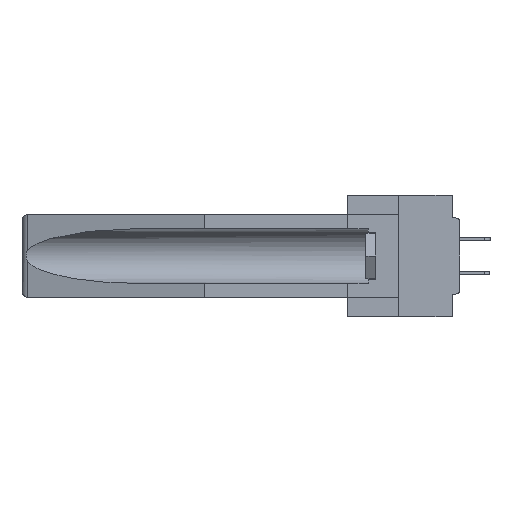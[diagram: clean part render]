
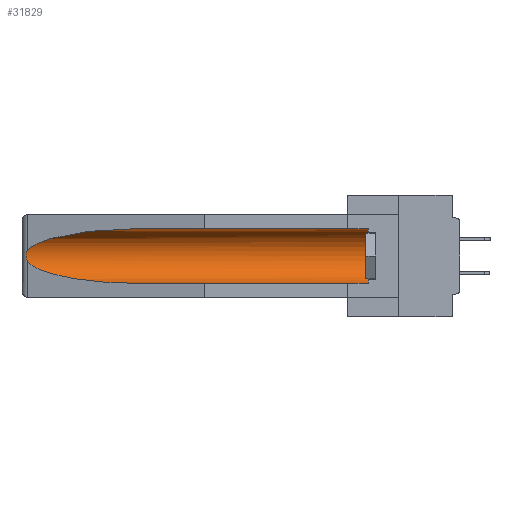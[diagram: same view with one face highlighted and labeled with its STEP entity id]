
A CAD part, left-side view. The second image highlights one B-rep face of the part: STEP entity #31829.
In plain terms, the highlighted cylindrical face has radius 2.857 mm (diameter 5.715 mm), a partial arc.
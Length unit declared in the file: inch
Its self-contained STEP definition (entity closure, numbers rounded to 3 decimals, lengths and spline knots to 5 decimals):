
#207 = VERTEX_POINT ( 'NONE', #28685 ) ;
#1543 = CARTESIAN_POINT ( 'NONE',  ( 0.155, -0.30754, -0.1715 ) ) ;
#2292 = EDGE_LOOP ( 'NONE', ( #20649, #12505, #21584, #20802, #36440, #23242 ) ) ;
#4876 = CARTESIAN_POINT ( 'NONE',  ( 0.26654, 1.53092, -0.15636 ) ) ;
#4993 = CARTESIAN_POINT ( 'NONE',  ( 0.26537, 1.52718, -0.19328 ) ) ;
#5123 = CARTESIAN_POINT ( 'NONE',  ( 0.26537, 1.52718, -0.14972 ) ) ;
#6769 = DIRECTION ( 'NONE',  ( 0., 1., 0. ) ) ;
#7559 = EDGE_CURVE ( 'NONE', #10433, #27864, #23436, .T. ) ;
#8415 = LINE ( 'NONE', #9465, #33361 ) ;
#8761 = CARTESIAN_POINT ( 'NONE',  ( 0.155, 0.126, -0.1715 ) ) ;
#8890 = VERTEX_POINT ( 'NONE', #21166 ) ;
#9349 = VECTOR ( 'NONE', #28162, 39.37008 ) ;
#9465 = CARTESIAN_POINT ( 'NONE',  ( 0.155, -0.30754, -0.284 ) ) ;
#9753 = CARTESIAN_POINT ( 'NONE',  ( 0.21114, 1.30732, -0.284 ) ) ;
#10433 = VERTEX_POINT ( 'NONE', #11585 ) ;
#10644 = CARTESIAN_POINT ( 'NONE',  ( 0.21114, 1.30732, -0.059 ) ) ;
#11585 = CARTESIAN_POINT ( 'NONE',  ( 0.155, 1.07973, -0.059 ) ) ;
#12113 = LINE ( 'NONE', #34651, #9349 ) ;
#12505 = ORIENTED_EDGE ( 'NONE', *, *, #20763, .T. ) ;
#12647 = CYLINDRICAL_SURFACE ( 'NONE', #29819, 0.1125 ) ;
#13329 = CARTESIAN_POINT ( 'NONE',  ( 0.155, 1.07973, -0.059 ) ) ;
#14302 = CARTESIAN_POINT ( 'NONE',  ( 0.155, 0.126, -0.059 ) ) ;
#15797 = VERTEX_POINT ( 'NONE', #14302 ) ;
#16316 = CARTESIAN_POINT ( 'NONE',  ( 0.2673, 1.53269, -0.17917 ) ) ;
#16463 = DIRECTION ( 'NONE',  ( 0., 0., 1. ) ) ;
#16539 =( BOUNDED_CURVE ( )  B_SPLINE_CURVE ( 3, ( #33118, #21356, #9753, #30893 ),
 .UNSPECIFIED., .F., .T. ) 
 B_SPLINE_CURVE_WITH_KNOTS ( ( 4, 4 ),
 ( 0.1948, 1.5708 ),
 .UNSPECIFIED. ) 
 CURVE ( )  GEOMETRIC_REPRESENTATION_ITEM ( )  RATIONAL_B_SPLINE_CURVE ( ( 1., 0.848, 0.848, 1. ) ) 
 REPRESENTATION_ITEM ( '' )  );
#16549 = CARTESIAN_POINT ( 'NONE',  ( 0.26537, 1.52718, -0.14972 ) ) ;
#16695 = CARTESIAN_POINT ( 'NONE',  ( 0.2675, 1.53308, -0.16763 ) ) ;
#17295 = EDGE_CURVE ( 'NONE', #207, #15797, #25272, .T. ) ;
#19099 = CARTESIAN_POINT ( 'NONE',  ( 0.26537, 1.52718, -0.14972 ) ) ;
#19664 = CARTESIAN_POINT ( 'NONE',  ( 0.26655, 1.53094, -0.18657 ) ) ;
#20649 = ORIENTED_EDGE ( 'NONE', *, *, #7559, .T. ) ;
#20763 = EDGE_CURVE ( 'NONE', #27864, #34786, #36192, .T. ) ;
#20802 = ORIENTED_EDGE ( 'NONE', *, *, #33819, .F. ) ;
#21166 = CARTESIAN_POINT ( 'NONE',  ( 0.155, 1.07973, -0.284 ) ) ;
#21356 = CARTESIAN_POINT ( 'NONE',  ( 0.25451, 1.48313, -0.24835 ) ) ;
#21584 = ORIENTED_EDGE ( 'NONE', *, *, #35502, .T. ) ;
#22172 = DIRECTION ( 'NONE',  ( 0., 1., 0. ) ) ;
#22521 = CARTESIAN_POINT ( 'NONE',  ( 0.26597, 1.52961, -0.15275 ) ) ;
#22653 = CARTESIAN_POINT ( 'NONE',  ( 0.2675, 1.53308, -0.17534 ) ) ;
#23242 = ORIENTED_EDGE ( 'NONE', *, *, #33519, .T. ) ;
#23436 =( BOUNDED_CURVE ( )  B_SPLINE_CURVE ( 3, ( #13329, #10644, #31288, #16549 ),
 .UNSPECIFIED., .F., .F. ) 
 B_SPLINE_CURVE_WITH_KNOTS ( ( 4, 4 ),
 ( 4.71239, 6.08839 ),
 .UNSPECIFIED. ) 
 CURVE ( )  GEOMETRIC_REPRESENTATION_ITEM ( )  RATIONAL_B_SPLINE_CURVE ( ( 1., 0.848, 0.848, 1. ) ) 
 REPRESENTATION_ITEM ( '' )  );
#23733 = CARTESIAN_POINT ( 'NONE',  ( 0.26537, 1.52718, -0.19328 ) ) ;
#25272 = CIRCLE ( 'NONE', #36651, 0.1125 ) ;
#25488 = CARTESIAN_POINT ( 'NONE',  ( 0.2673, 1.5327, -0.16383 ) ) ;
#25619 = CARTESIAN_POINT ( 'NONE',  ( 0.26597, 1.5296, -0.19026 ) ) ;
#26684 = DIRECTION ( 'NONE',  ( 0., 0., 1. ) ) ;
#27864 = VERTEX_POINT ( 'NONE', #19099 ) ;
#28162 = DIRECTION ( 'NONE',  ( 0., 1., 0. ) ) ;
#28324 = FACE_OUTER_BOUND ( 'NONE', #2292, .T. ) ;
#28685 = CARTESIAN_POINT ( 'NONE',  ( 0.155, 0.126, -0.284 ) ) ;
#29382 = DIRECTION ( 'NONE',  ( 0., -1., 0. ) ) ;
#29819 = AXIS2_PLACEMENT_3D ( 'NONE', #1543, #22172, #16463 ) ;
#30893 = CARTESIAN_POINT ( 'NONE',  ( 0.155, 1.07973, -0.284 ) ) ;
#31288 = CARTESIAN_POINT ( 'NONE',  ( 0.25451, 1.48313, -0.09465 ) ) ;
#31829 = ADVANCED_FACE ( 'NONE', ( #28324 ), #12647, .F. ) ;
#33118 = CARTESIAN_POINT ( 'NONE',  ( 0.26537, 1.52718, -0.19328 ) ) ;
#33361 = VECTOR ( 'NONE', #6769, 39.37008 ) ;
#33519 = EDGE_CURVE ( 'NONE', #15797, #10433, #12113, .T. ) ;
#33819 = EDGE_CURVE ( 'NONE', #207, #8890, #8415, .T. ) ;
#34651 = CARTESIAN_POINT ( 'NONE',  ( 0.155, -0.30754, -0.059 ) ) ;
#34786 = VERTEX_POINT ( 'NONE', #23733 ) ;
#35502 = EDGE_CURVE ( 'NONE', #34786, #8890, #16539, .T. ) ;
#36192 = B_SPLINE_CURVE_WITH_KNOTS ( 'NONE', 3,
 ( #5123, #22521, #4876, #25488, #16695, #22653, #16316, #19664, #25619, #4993 ),
 .UNSPECIFIED., .F., .F.,
 ( 4, 2, 2, 2, 4 ),
 ( 0., 0.00029, 0.00058, 0.00087, 0.00117 ),
 .UNSPECIFIED. ) ;
#36440 = ORIENTED_EDGE ( 'NONE', *, *, #17295, .T. ) ;
#36651 = AXIS2_PLACEMENT_3D ( 'NONE', #8761, #29382, #26684 ) ;
